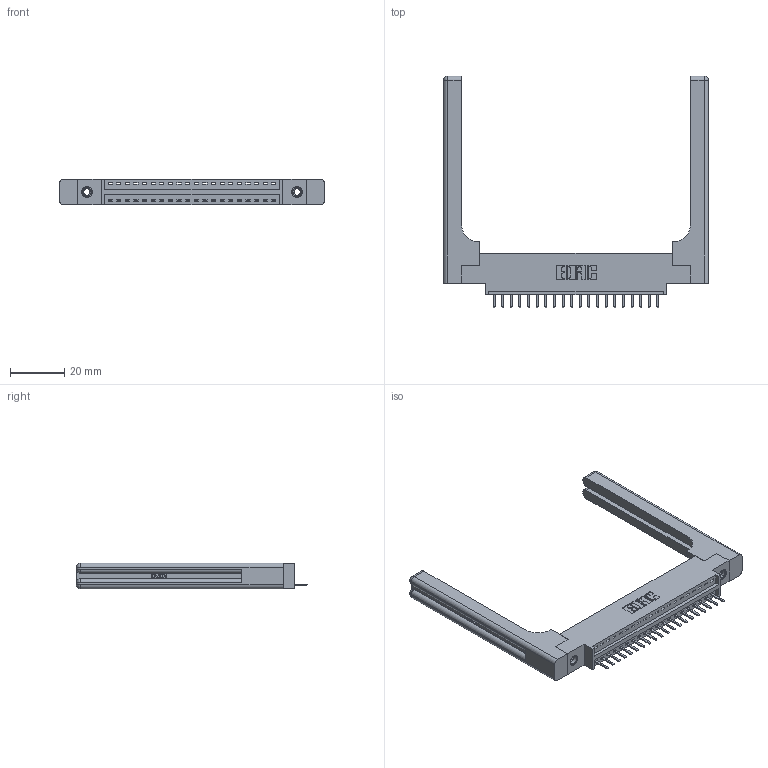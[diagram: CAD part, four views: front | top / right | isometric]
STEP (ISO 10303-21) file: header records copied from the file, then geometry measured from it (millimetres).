
FILE_DESCRIPTION (( 'STEP AP203' ), '1' );
FILE_NAME ('396-020-520-658.STEP', '2019-10-26T21:09:25', ( '' ), ( '' ), 'SwSTEP 2.0', 'SolidWorks 2016', '' );
FILE_SCHEMA (( 'CONFIG_CONTROL_DESIGN' ));
Length unit declared in the file: inch
Products named in the file (5): 346 Part_0.170 Offset - 0.156 Dia-TH; 345-292-001_345-293-120; 396-020-520-658; 346-220-058_345-220-058; 345-250-001_345-250-001-102
Assembly tree (25 placements, depth 2):
  396-020-520-658
    346 Part_0.170 Offset - 0.156 Dia-TH
    345-292-001_345-293-120  x20
    345-250-001_345-250-001-102  x2
    346-220-058_345-220-058  x2
Bounding box: 97.56 x 85.29 x 9.4 mm (x, y, z)
Volume: 16493.5 mm3; surface area: 16118.1 mm2
Topology: 25 solids, 25 shells, 1622 faces, 4687 edges, 3050 vertices
Faces by surface type: plane 1068, cylinder 494, bspline 36, cone 12, sphere 8, torus 4
Entity records: 20802 total; most frequent: CARTESIAN_POINT 4565, ORIENTED_EDGE 3304, DIRECTION 2972, EDGE_CURVE 1652, VECTOR 1344, LINE 1344, VERTEX_POINT 1090, AXIS2_PLACEMENT_3D 814
